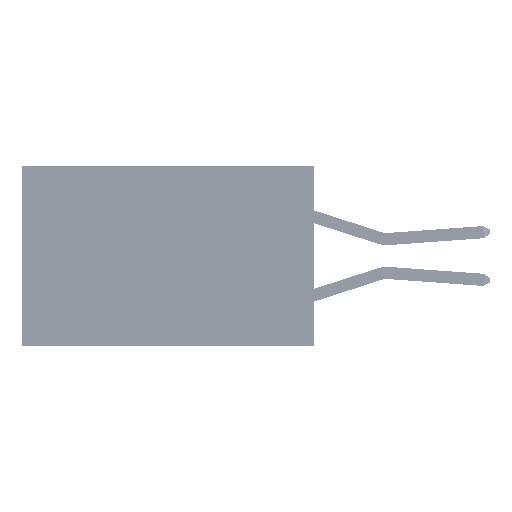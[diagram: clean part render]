
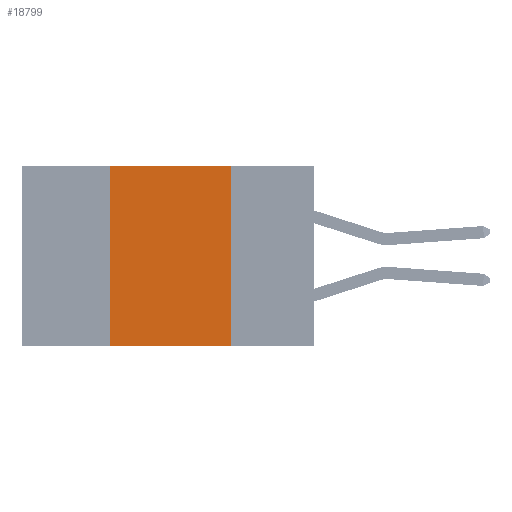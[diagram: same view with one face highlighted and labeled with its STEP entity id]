
A CAD part, left-side view. The second image highlights one B-rep face of the part: STEP entity #18799.
In plain terms, the highlighted planar face has unit normal (-1, 0, 0).
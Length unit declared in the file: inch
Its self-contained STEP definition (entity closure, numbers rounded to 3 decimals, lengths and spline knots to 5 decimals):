
#661 = CARTESIAN_POINT ( 'NONE',  ( 0., 0.6, -0.37 ) ) ;
#2627 = VERTEX_POINT ( 'NONE', #29977 ) ;
#2850 = LINE ( 'NONE', #4244, #18086 ) ;
#4244 = CARTESIAN_POINT ( 'NONE',  ( 0., 0.42, 0. ) ) ;
#4625 = ORIENTED_EDGE ( 'NONE', *, *, #47771, .F. ) ;
#4973 = FACE_OUTER_BOUND ( 'NONE', #19276, .T. ) ;
#8069 = LINE ( 'NONE', #30310, #25865 ) ;
#10365 = ORIENTED_EDGE ( 'NONE', *, *, #15922, .F. ) ;
#10917 = VECTOR ( 'NONE', #14391, 39.37008 ) ;
#12717 = DIRECTION ( 'NONE',  ( 0., 0., 1. ) ) ;
#14391 = DIRECTION ( 'NONE',  ( 0., 0., -1. ) ) ;
#14437 = ORIENTED_EDGE ( 'NONE', *, *, #18659, .T. ) ;
#14562 = EDGE_CURVE ( 'NONE', #43918, #2627, #2850, .T. ) ;
#14729 = VERTEX_POINT ( 'NONE', #17513 ) ;
#15922 = EDGE_CURVE ( 'NONE', #23650, #14729, #21751, .T. ) ;
#17430 = AXIS2_PLACEMENT_3D ( 'NONE', #50693, #46581, #42165 ) ;
#17513 = CARTESIAN_POINT ( 'NONE',  ( 0., 0.17, -0.37 ) ) ;
#18086 = VECTOR ( 'NONE', #12717, 39.37008 ) ;
#18659 = EDGE_CURVE ( 'NONE', #43918, #14729, #27154, .T. ) ;
#18799 = ADVANCED_FACE ( 'NONE', ( #4973 ), #50162, .F. ) ;
#19276 = EDGE_LOOP ( 'NONE', ( #10365, #4625, #23558, #14437 ) ) ;
#21751 = LINE ( 'NONE', #26139, #10917 ) ;
#22151 = DIRECTION ( 'NONE',  ( 0., -1., 0. ) ) ;
#23558 = ORIENTED_EDGE ( 'NONE', *, *, #14562, .F. ) ;
#23650 = VERTEX_POINT ( 'NONE', #50293 ) ;
#25865 = VECTOR ( 'NONE', #22151, 39.37008 ) ;
#26139 = CARTESIAN_POINT ( 'NONE',  ( 0., 0.17, 0. ) ) ;
#27154 = LINE ( 'NONE', #661, #46178 ) ;
#29977 = CARTESIAN_POINT ( 'NONE',  ( 0., 0.42, 0. ) ) ;
#30310 = CARTESIAN_POINT ( 'NONE',  ( 0., 0.6, 0. ) ) ;
#31209 = CARTESIAN_POINT ( 'NONE',  ( 0., 0.42, -0.37 ) ) ;
#42165 = DIRECTION ( 'NONE',  ( 0., 0., -1. ) ) ;
#43918 = VERTEX_POINT ( 'NONE', #31209 ) ;
#46178 = VECTOR ( 'NONE', #49289, 39.37008 ) ;
#46581 = DIRECTION ( 'NONE',  ( 1., 0., 0. ) ) ;
#47771 = EDGE_CURVE ( 'NONE', #2627, #23650, #8069, .T. ) ;
#49289 = DIRECTION ( 'NONE',  ( 0., -1., 0. ) ) ;
#50162 = PLANE ( 'NONE',  #17430 ) ;
#50293 = CARTESIAN_POINT ( 'NONE',  ( 0., 0.17, 0. ) ) ;
#50693 = CARTESIAN_POINT ( 'NONE',  ( 0., 0.6, 0. ) ) ;
